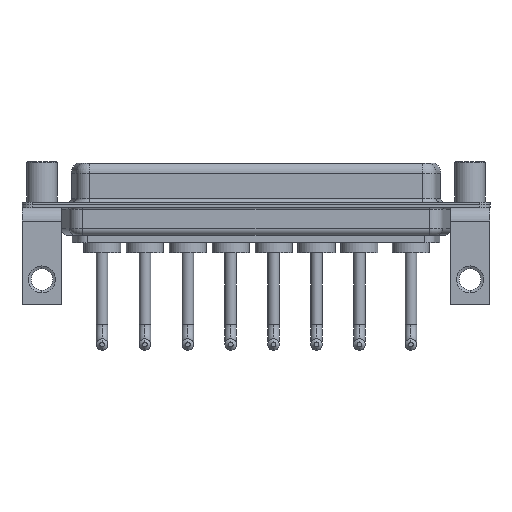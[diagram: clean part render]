
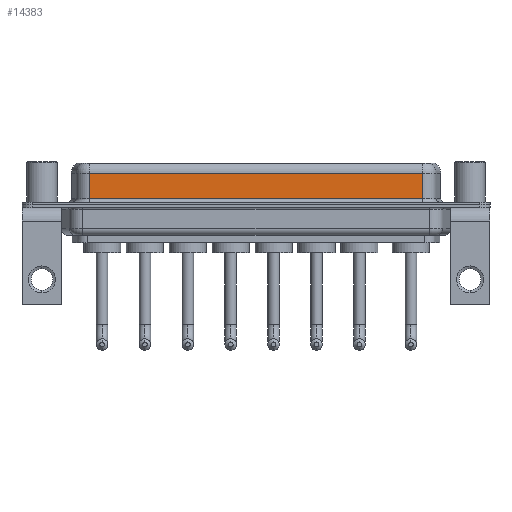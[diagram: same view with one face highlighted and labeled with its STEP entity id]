
A CAD part, front view. The second image highlights one B-rep face of the part: STEP entity #14383.
In plain terms, the highlighted planar face has unit normal (0, -1, 0).
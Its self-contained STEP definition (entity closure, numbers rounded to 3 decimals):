
#438 = EDGE_CURVE ( 'NONE', #937, #10645, #4432, .T. ) ;
#937 = VERTEX_POINT ( 'NONE', #6733 ) ;
#2273 = VECTOR ( 'NONE', #13309, 1000. ) ;
#2647 = VECTOR ( 'NONE', #10257, 1000. ) ;
#3984 = VERTEX_POINT ( 'NONE', #15694 ) ;
#4432 = LINE ( 'NONE', #9314, #2647 ) ;
#4727 = DIRECTION ( 'NONE',  ( 1., 0., 0. ) ) ;
#4772 = DIRECTION ( 'NONE',  ( 0., 0., -1. ) ) ;
#4907 = EDGE_CURVE ( 'NONE', #3984, #6153, #12120, .T. ) ;
#5086 = ORIENTED_EDGE ( 'NONE', *, *, #438, .T. ) ;
#5339 = EDGE_CURVE ( 'NONE', #3984, #937, #15772, .T. ) ;
#5387 = ORIENTED_EDGE ( 'NONE', *, *, #4907, .F. ) ;
#5400 = FACE_OUTER_BOUND ( 'NONE', #6575, .T. ) ;
#6153 = VERTEX_POINT ( 'NONE', #12094 ) ;
#6575 = EDGE_LOOP ( 'NONE', ( #5387, #14342, #5086, #14641 ) ) ;
#6733 = CARTESIAN_POINT ( 'NONE',  ( 7.038, -3.95, 4.65 ) ) ;
#9083 = DIRECTION ( 'NONE',  ( 0., 1., 0. ) ) ;
#9314 = CARTESIAN_POINT ( 'NONE',  ( 7.038, -3.95, 6.4 ) ) ;
#9726 = CARTESIAN_POINT ( 'NONE',  ( 56.462, -3.95, 6.4 ) ) ;
#10257 = DIRECTION ( 'NONE',  ( 0., 0., -1. ) ) ;
#10269 = PLANE ( 'NONE',  #13642 ) ;
#10397 = EDGE_CURVE ( 'NONE', #10645, #6153, #10786, .T. ) ;
#10645 = VERTEX_POINT ( 'NONE', #10689 ) ;
#10689 = CARTESIAN_POINT ( 'NONE',  ( 7.038, -3.95, 0.9 ) ) ;
#10786 = LINE ( 'NONE', #15667, #14618 ) ;
#12094 = CARTESIAN_POINT ( 'NONE',  ( 56.462, -3.95, 0.9 ) ) ;
#12120 = LINE ( 'NONE', #9726, #15790 ) ;
#13309 = DIRECTION ( 'NONE',  ( -1., 0., 0. ) ) ;
#13642 = AXIS2_PLACEMENT_3D ( 'NONE', #15153, #9083, #13963 ) ;
#13963 = DIRECTION ( 'NONE',  ( 0., 0., 1. ) ) ;
#14342 = ORIENTED_EDGE ( 'NONE', *, *, #5339, .T. ) ;
#14383 = ADVANCED_FACE ( 'NONE', ( #5400 ), #10269, .F. ) ;
#14513 = CARTESIAN_POINT ( 'NONE',  ( 56.462, -3.95, 4.65 ) ) ;
#14618 = VECTOR ( 'NONE', #4727, 1000. ) ;
#14641 = ORIENTED_EDGE ( 'NONE', *, *, #10397, .T. ) ;
#15153 = CARTESIAN_POINT ( 'NONE',  ( 56.462, -3.95, 6.4 ) ) ;
#15667 = CARTESIAN_POINT ( 'NONE',  ( 56.462, -3.95, 0.9 ) ) ;
#15694 = CARTESIAN_POINT ( 'NONE',  ( 56.462, -3.95, 4.65 ) ) ;
#15772 = LINE ( 'NONE', #14513, #2273 ) ;
#15790 = VECTOR ( 'NONE', #4772, 1000. ) ;
